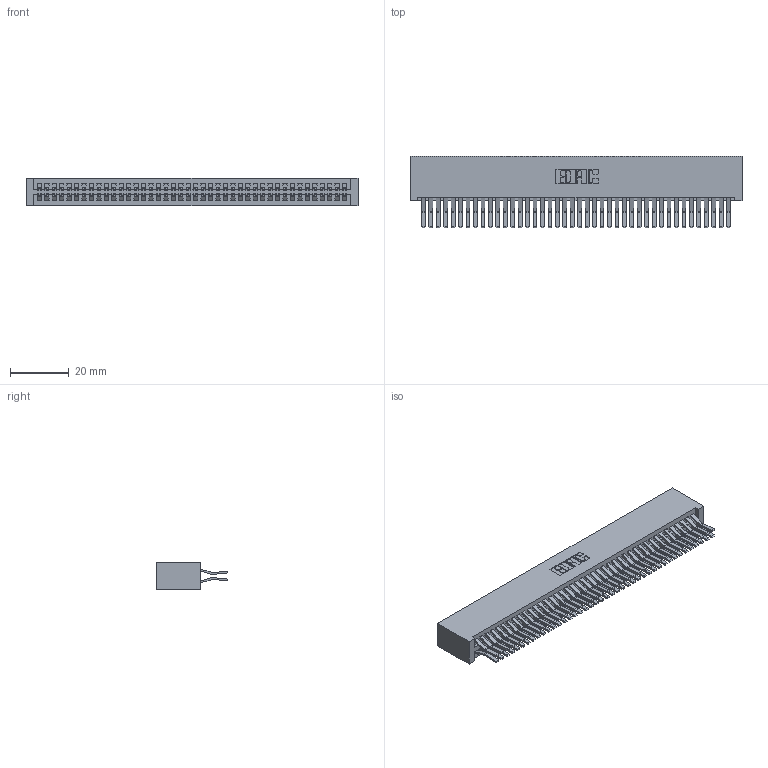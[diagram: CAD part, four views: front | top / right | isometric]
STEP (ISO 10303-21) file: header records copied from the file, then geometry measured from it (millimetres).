
FILE_DESCRIPTION (( 'STEP AP203' ), '1' );
FILE_NAME ('345-084-560-201.STEP', '2019-11-01T05:56:49', ( '' ), ( '' ), 'SwSTEP 2.0', 'SolidWorks 2016', '' );
FILE_SCHEMA (( 'CONFIG_CONTROL_DESIGN' ));
Length unit declared in the file: inch
Products named in the file (3): 345-084-560-201; 345 Part_No Mounting Lugs; 345-292-001_560 Tail
Assembly tree (85 placements, depth 2):
  345-084-560-201
    345 Part_No Mounting Lugs
    345-292-001_560 Tail  x84
Bounding box: 113.28 x 24.45 x 9.4 mm (x, y, z)
Volume: 12171 mm3; surface area: 19710.1 mm2
Topology: 85 solids, 85 shells, 4486 faces, 13337 edges, 8778 vertices
Faces by surface type: plane 2848, cylinder 1638
Entity records: 32765 total; most frequent: CARTESIAN_POINT 5492, ORIENTED_EDGE 5426, DIRECTION 4841, EDGE_CURVE 2713, VECTOR 2417, LINE 2417, VERTEX_POINT 1806, AXIS2_PLACEMENT_3D 1212
